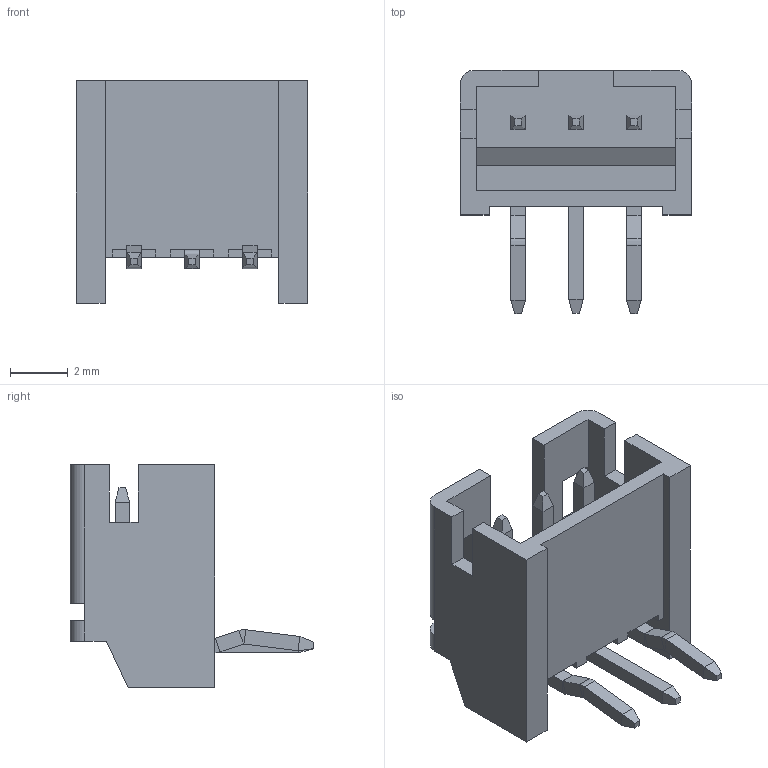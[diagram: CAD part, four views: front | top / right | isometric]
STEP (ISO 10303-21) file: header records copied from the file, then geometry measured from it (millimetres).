
FILE_DESCRIPTION (( 'STEP AP203' ), '1' );
FILE_NAME ('140-503-415-000.STEP', '2020-03-31T19:40:36', ( '' ), ( '' ), 'SwSTEP 2.0', 'SolidWorks 2016', '' );
FILE_SCHEMA (( 'CONFIG_CONTROL_DESIGN' ));
Length unit declared in the file: millimetre
Products named in the file (4): 140-503-415-000; RA Contact_Kink; RA Housing_503; RA Contact_Str
Assembly tree (4 placements, depth 2):
  140-503-415-000
    RA Housing_503
    RA Contact_Kink  x2
    RA Contact_Str
Bounding box: 8 x 8.41 x 7.7 mm (x, y, z)
Volume: 118.9 mm3; surface area: 429.1 mm2
Topology: 4 solids, 4 shells, 169 faces, 405 edges, 242 vertices
Faces by surface type: plane 151, cylinder 18
Entity records: 4257 total; most frequent: CARTESIAN_POINT 669, ORIENTED_EDGE 658, DIRECTION 629, EDGE_CURVE 329, LINE 305, VECTOR 305, VERTEX_POINT 202, AXIS2_PLACEMENT_3D 162
